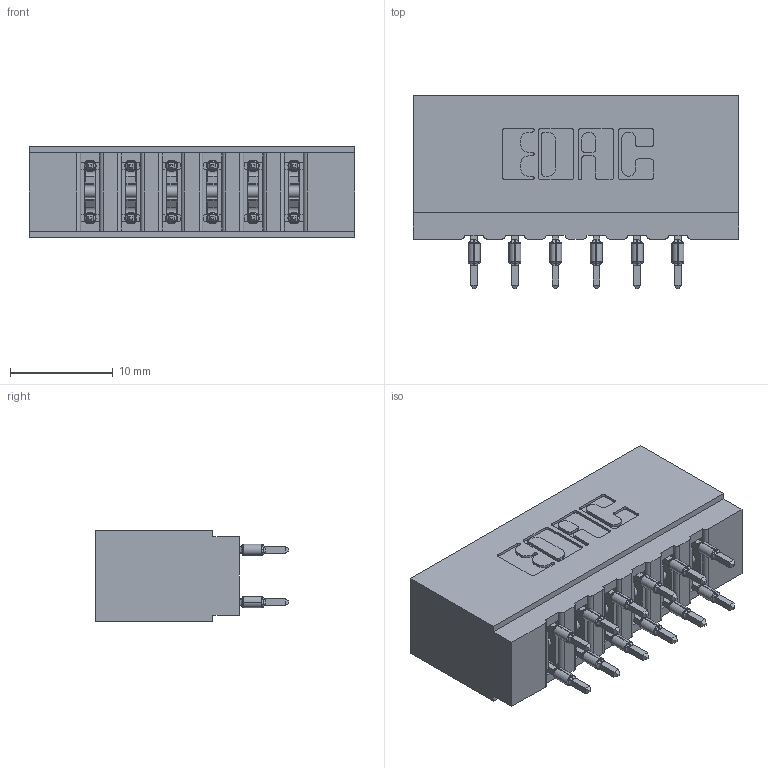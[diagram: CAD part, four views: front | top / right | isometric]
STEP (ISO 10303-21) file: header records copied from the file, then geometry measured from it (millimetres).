
FILE_DESCRIPTION (( 'STEP AP203' ), '1' );
FILE_NAME ('717-012-560-201.STEP', '2026-02-20T17:00:39', ( '' ), ( '' ), 'SwSTEP 2.0', 'SolidWorks 2023', '' );
FILE_SCHEMA (( 'CONFIG_CONTROL_DESIGN' ));
Length unit declared in the file: millimetre
Products named in the file (3): 717-012-560-201; 745-292-001_560; 717 Part_Insulator Option - 06
Assembly tree (13 placements, depth 2):
  717-012-560-201
    717 Part_Insulator Option - 06
    745-292-001_560  x12
Bounding box: 31.65 x 18.78 x 8.89 mm (x, y, z)
Volume: 2935.6 mm3; surface area: 4218.3 mm2
Topology: 13 solids, 13 shells, 1282 faces, 3503 edges, 2230 vertices
Faces by surface type: plane 672, cylinder 298, bspline 240, torus 72
Entity records: 15468 total; most frequent: CARTESIAN_POINT 3199, ORIENTED_EDGE 2562, DIRECTION 2275, EDGE_CURVE 1281, VECTOR 1055, LINE 1055, VERTEX_POINT 822, AXIS2_PLACEMENT_3D 610
